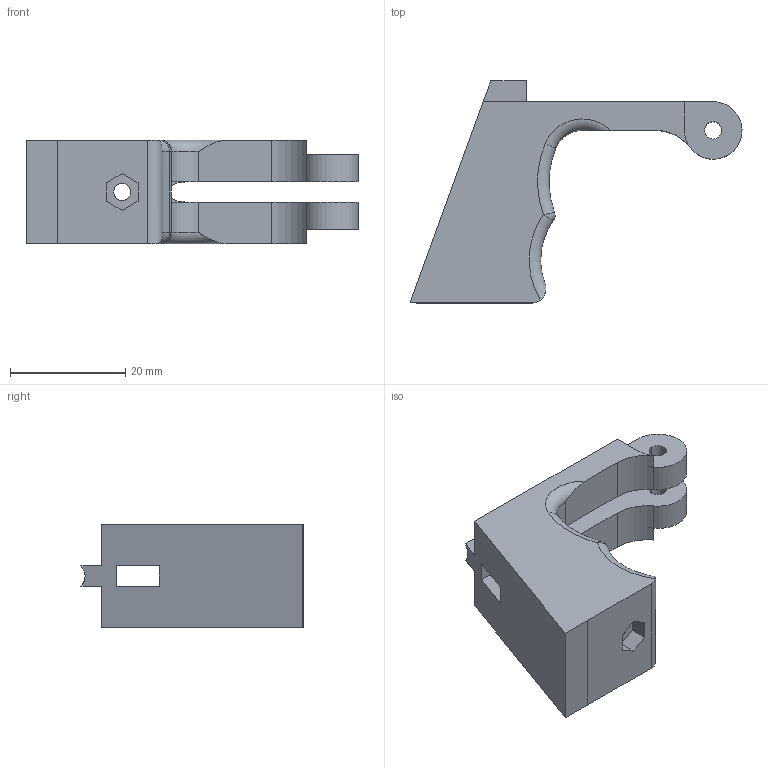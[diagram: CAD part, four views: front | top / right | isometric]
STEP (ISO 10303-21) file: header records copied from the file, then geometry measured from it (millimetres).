
FILE_DESCRIPTION (( 'STEP AP214' ), '1' );
FILE_NAME ('Grip^Launcher2_1.STEP', '2014-10-07T00:03:41', ( 'WarFairy' ), ( '' ), 'SwSTEP 2.0', 'SolidWorks 2013', '' );
FILE_SCHEMA (( 'AUTOMOTIVE_DESIGN' ));
Length unit declared in the file: millimetre
Products named in the file (1): Grip^Launcher2_1
Bounding box: 57.72 x 38.63 x 18 mm (x, y, z)
Volume: 13061.2 mm3; surface area: 5504.2 mm2
Topology: 1 solids, 1 shells, 57 faces, 157 edges, 100 vertices
Faces by surface type: plane 26, cylinder 23, torus 6, bspline 2
Entity records: 2097 total; most frequent: CARTESIAN_POINT 585, ORIENTED_EDGE 310, DIRECTION 309, EDGE_CURVE 155, AXIS2_PLACEMENT_3D 109, VERTEX_POINT 100, VECTOR 91, LINE 91
